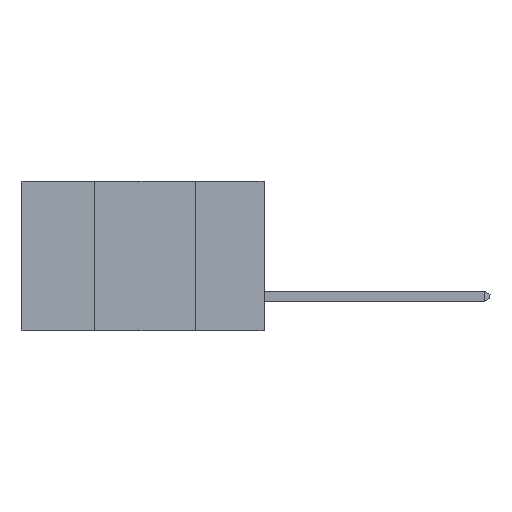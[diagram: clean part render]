
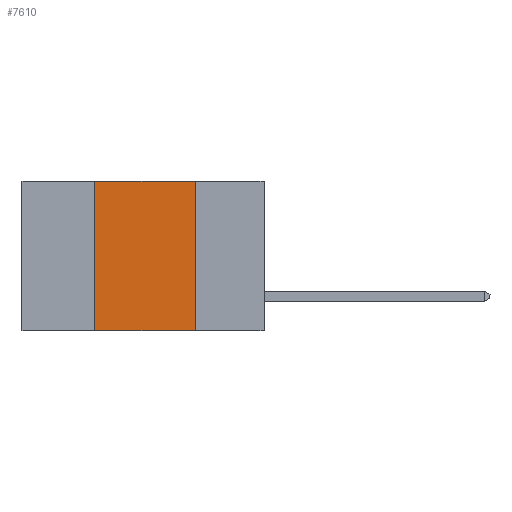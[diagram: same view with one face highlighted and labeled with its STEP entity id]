
A CAD part, left-side view. The second image highlights one B-rep face of the part: STEP entity #7610.
In plain terms, the highlighted planar face has unit normal (-1, 0, 0).
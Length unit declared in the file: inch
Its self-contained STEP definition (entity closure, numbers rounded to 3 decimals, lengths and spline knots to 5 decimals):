
#263 = VERTEX_POINT ( 'NONE', #6020 ) ;
#546 = CARTESIAN_POINT ( 'NONE',  ( 0., 0.17, -0.37 ) ) ;
#610 = DIRECTION ( 'NONE',  ( 0., -1., 0. ) ) ;
#880 = DIRECTION ( 'NONE',  ( 0., 0., -1. ) ) ;
#1357 = CARTESIAN_POINT ( 'NONE',  ( 0., 0.6, -0.37 ) ) ;
#1360 = EDGE_CURVE ( 'NONE', #2943, #8304, #1621, .T. ) ;
#1364 = CARTESIAN_POINT ( 'NONE',  ( 0., 0.42, -0.37 ) ) ;
#1621 = LINE ( 'NONE', #546, #2154 ) ;
#1756 = LINE ( 'NONE', #4545, #3505 ) ;
#2015 = ORIENTED_EDGE ( 'NONE', *, *, #1360, .F. ) ;
#2154 = VECTOR ( 'NONE', #880, 39.37008 ) ;
#2182 = EDGE_LOOP ( 'NONE', ( #2015, #3053, #7399, #7401 ) ) ;
#2382 = CARTESIAN_POINT ( 'NONE',  ( 0., 0.42, -0.37 ) ) ;
#2702 = CARTESIAN_POINT ( 'NONE',  ( 0., 0.17, 0. ) ) ;
#2943 = VERTEX_POINT ( 'NONE', #2702 ) ;
#3053 = ORIENTED_EDGE ( 'NONE', *, *, #6349, .F. ) ;
#3505 = VECTOR ( 'NONE', #6110, 39.37008 ) ;
#4024 = DIRECTION ( 'NONE',  ( 0., 0., -1. ) ) ;
#4351 = DIRECTION ( 'NONE',  ( 0., 0., 1. ) ) ;
#4538 = LINE ( 'NONE', #1357, #4733 ) ;
#4545 = CARTESIAN_POINT ( 'NONE',  ( 0., 0.6, 0. ) ) ;
#4656 = CARTESIAN_POINT ( 'NONE',  ( 0., 0.6, 0. ) ) ;
#4733 = VECTOR ( 'NONE', #610, 39.37008 ) ;
#4798 = FACE_OUTER_BOUND ( 'NONE', #2182, .T. ) ;
#5176 = CARTESIAN_POINT ( 'NONE',  ( 0., 0.17, -0.37 ) ) ;
#6020 = CARTESIAN_POINT ( 'NONE',  ( 0., 0.42, 0. ) ) ;
#6110 = DIRECTION ( 'NONE',  ( 0., -1., 0. ) ) ;
#6315 = DIRECTION ( 'NONE',  ( 1., 0., 0. ) ) ;
#6349 = EDGE_CURVE ( 'NONE', #263, #2943, #1756, .T. ) ;
#6941 = AXIS2_PLACEMENT_3D ( 'NONE', #4656, #6315, #4024 ) ;
#7146 = LINE ( 'NONE', #1364, #8478 ) ;
#7399 = ORIENTED_EDGE ( 'NONE', *, *, #7746, .F. ) ;
#7401 = ORIENTED_EDGE ( 'NONE', *, *, #8293, .T. ) ;
#7610 = ADVANCED_FACE ( 'NONE', ( #4798 ), #8474, .F. ) ;
#7746 = EDGE_CURVE ( 'NONE', #8377, #263, #7146, .T. ) ;
#8293 = EDGE_CURVE ( 'NONE', #8377, #8304, #4538, .T. ) ;
#8304 = VERTEX_POINT ( 'NONE', #5176 ) ;
#8377 = VERTEX_POINT ( 'NONE', #2382 ) ;
#8474 = PLANE ( 'NONE',  #6941 ) ;
#8478 = VECTOR ( 'NONE', #4351, 39.37008 ) ;
